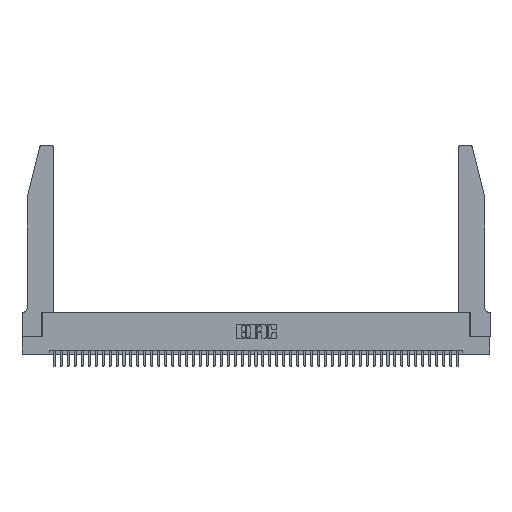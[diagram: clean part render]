
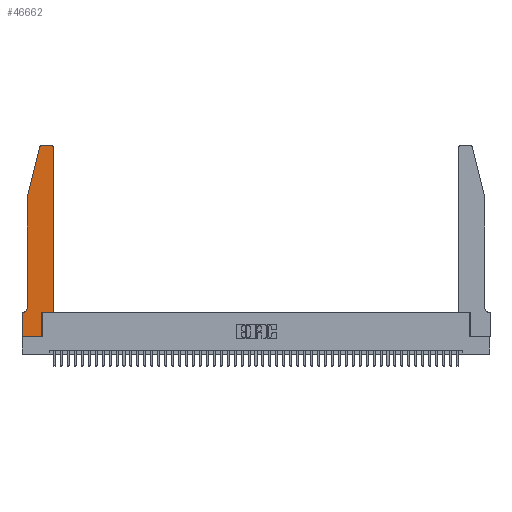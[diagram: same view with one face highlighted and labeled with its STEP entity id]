
A CAD part, top view. The second image highlights one B-rep face of the part: STEP entity #46662.
In plain terms, the highlighted planar face has unit normal (0, 0, 1).
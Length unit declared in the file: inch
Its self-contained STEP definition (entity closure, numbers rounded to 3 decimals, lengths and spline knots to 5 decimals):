
#1175 = AXIS2_PLACEMENT_3D ( 'NONE', #30477, #7696, #34262 ) ;
#1360 = EDGE_CURVE ( 'NONE', #37964, #4641, #27871, .T. ) ;
#1802 = VERTEX_POINT ( 'NONE', #13973 ) ;
#1859 = CARTESIAN_POINT ( 'NONE',  ( 0.0755, 2., 0.37 ) ) ;
#1992 = CARTESIAN_POINT ( 'NONE',  ( 0., 0., 0.37 ) ) ;
#2021 = DIRECTION ( 'NONE',  ( 0., 1., 0. ) ) ;
#2385 = DIRECTION ( 'NONE',  ( 0., -1., 0. ) ) ;
#2411 = EDGE_LOOP ( 'NONE', ( #35080, #6524, #41640, #19693, #6158, #15713, #20523, #47466, #19174, #46541, #48551, #15309 ) ) ;
#4641 = VERTEX_POINT ( 'NONE', #20457 ) ;
#5832 = CARTESIAN_POINT ( 'NONE',  ( 0.2865, 0.35, 0.37 ) ) ;
#6158 = ORIENTED_EDGE ( 'NONE', *, *, #45871, .T. ) ;
#6491 = VERTEX_POINT ( 'NONE', #12283 ) ;
#6518 = CARTESIAN_POINT ( 'NONE',  ( 0.2865, 0., 0.37 ) ) ;
#6524 = ORIENTED_EDGE ( 'NONE', *, *, #12069, .T. ) ;
#6620 = CIRCLE ( 'NONE', #1175, 0.07 ) ;
#7099 = CIRCLE ( 'NONE', #15949, 0.03 ) ;
#7696 = DIRECTION ( 'NONE',  ( 0., 0., -1. ) ) ;
#8002 = EDGE_CURVE ( 'NONE', #47248, #38260, #21926, .T. ) ;
#8680 = CARTESIAN_POINT ( 'NONE',  ( 0.25487, 2.72718, 0.37 ) ) ;
#8787 = LINE ( 'NONE', #15213, #39152 ) ;
#9561 = DIRECTION ( 'NONE',  ( 0., 0., 1. ) ) ;
#11467 = VERTEX_POINT ( 'NONE', #20448 ) ;
#12069 = EDGE_CURVE ( 'NONE', #30801, #13946, #47593, .T. ) ;
#12283 = CARTESIAN_POINT ( 'NONE',  ( 0.4205, 2.75, 0.37 ) ) ;
#12477 = CARTESIAN_POINT ( 'NONE',  ( 0.4205, 2.72, 0.37 ) ) ;
#13946 = VERTEX_POINT ( 'NONE', #8680 ) ;
#13973 = CARTESIAN_POINT ( 'NONE',  ( 0., 0.35, 0.37 ) ) ;
#14581 = AXIS2_PLACEMENT_3D ( 'NONE', #16002, #46081, #23686 ) ;
#14727 = LINE ( 'NONE', #1859, #43635 ) ;
#15213 = CARTESIAN_POINT ( 'NONE',  ( 0.2605, 2.75, 0.37 ) ) ;
#15309 = ORIENTED_EDGE ( 'NONE', *, *, #34329, .T. ) ;
#15360 = EDGE_CURVE ( 'NONE', #4641, #11467, #21247, .T. ) ;
#15378 = VERTEX_POINT ( 'NONE', #26697 ) ;
#15713 = ORIENTED_EDGE ( 'NONE', *, *, #29901, .T. ) ;
#15949 = AXIS2_PLACEMENT_3D ( 'NONE', #12477, #38962, #16351 ) ;
#16002 = CARTESIAN_POINT ( 'NONE',  ( 0., 0.35, 0.37 ) ) ;
#16351 = DIRECTION ( 'NONE',  ( 1., 0., 0. ) ) ;
#17013 = DIRECTION ( 'NONE',  ( -0.239, -0.971, 0. ) ) ;
#18178 = VERTEX_POINT ( 'NONE', #44987 ) ;
#18852 = DIRECTION ( 'NONE',  ( 0., 1., 0. ) ) ;
#19037 = DIRECTION ( 'NONE',  ( -1., 0., 0. ) ) ;
#19174 = ORIENTED_EDGE ( 'NONE', *, *, #48269, .T. ) ;
#19693 = ORIENTED_EDGE ( 'NONE', *, *, #43758, .T. ) ;
#20448 = CARTESIAN_POINT ( 'NONE',  ( 0.4505, 2.72, 0.37 ) ) ;
#20457 = CARTESIAN_POINT ( 'NONE',  ( 0.4505, 0.35, 0.37 ) ) ;
#20523 = ORIENTED_EDGE ( 'NONE', *, *, #46788, .T. ) ;
#20741 = VECTOR ( 'NONE', #36001, 39.37008 ) ;
#21167 = FACE_OUTER_BOUND ( 'NONE', #2411, .T. ) ;
#21247 = LINE ( 'NONE', #37838, #31309 ) ;
#21910 = CARTESIAN_POINT ( 'NONE',  ( 0.0755, 0.35, 0.37 ) ) ;
#21926 = LINE ( 'NONE', #1992, #20741 ) ;
#23614 = LINE ( 'NONE', #43894, #32454 ) ;
#23686 = DIRECTION ( 'NONE',  ( 1., 0., 0. ) ) ;
#24168 = CARTESIAN_POINT ( 'NONE',  ( 0., 0., 0.37 ) ) ;
#24680 = CARTESIAN_POINT ( 'NONE',  ( 0.0755, 0.42, 0.37 ) ) ;
#24793 = VECTOR ( 'NONE', #40813, 39.37008 ) ;
#25909 = AXIS2_PLACEMENT_3D ( 'NONE', #32343, #9561, #36102 ) ;
#26522 = LINE ( 'NONE', #24168, #46381 ) ;
#26685 = VECTOR ( 'NONE', #38451, 39.37008 ) ;
#26697 = CARTESIAN_POINT ( 'NONE',  ( 0.0755, 2., 0.37 ) ) ;
#27871 = LINE ( 'NONE', #30909, #26685 ) ;
#29475 = LINE ( 'NONE', #21910, #24793 ) ;
#29901 = EDGE_CURVE ( 'NONE', #18178, #1802, #29475, .T. ) ;
#30477 = CARTESIAN_POINT ( 'NONE',  ( 0.0055, 0.42, 0.37 ) ) ;
#30801 = VERTEX_POINT ( 'NONE', #31080 ) ;
#30909 = CARTESIAN_POINT ( 'NONE',  ( 0.4505, 0.35, 0.37 ) ) ;
#31080 = CARTESIAN_POINT ( 'NONE',  ( 0.284, 2.75, 0.37 ) ) ;
#31309 = VECTOR ( 'NONE', #18852, 39.37008 ) ;
#31566 = DIRECTION ( 'NONE',  ( 0., -1., 0. ) ) ;
#31655 = LINE ( 'NONE', #5832, #40444 ) ;
#32343 = CARTESIAN_POINT ( 'NONE',  ( 0.284, 2.72, 0.37 ) ) ;
#32454 = VECTOR ( 'NONE', #2385, 39.37008 ) ;
#32978 = EDGE_CURVE ( 'NONE', #6491, #30801, #8787, .T. ) ;
#33901 = VERTEX_POINT ( 'NONE', #24680 ) ;
#34262 = DIRECTION ( 'NONE',  ( -1., 0., 0. ) ) ;
#34329 = EDGE_CURVE ( 'NONE', #11467, #6491, #7099, .T. ) ;
#35080 = ORIENTED_EDGE ( 'NONE', *, *, #32978, .T. ) ;
#36001 = DIRECTION ( 'NONE',  ( 1., 0., 0. ) ) ;
#36102 = DIRECTION ( 'NONE',  ( 1., 0., 0. ) ) ;
#36408 = EDGE_CURVE ( 'NONE', #13946, #15378, #14727, .T. ) ;
#37838 = CARTESIAN_POINT ( 'NONE',  ( 0.4505, 0.35, 0.37 ) ) ;
#37964 = VERTEX_POINT ( 'NONE', #42455 ) ;
#38067 = CARTESIAN_POINT ( 'NONE',  ( 0., 0., 0.37 ) ) ;
#38260 = VERTEX_POINT ( 'NONE', #6518 ) ;
#38451 = DIRECTION ( 'NONE',  ( 1., 0., 0. ) ) ;
#38618 = PLANE ( 'NONE',  #14581 ) ;
#38962 = DIRECTION ( 'NONE',  ( 0., 0., 1. ) ) ;
#39152 = VECTOR ( 'NONE', #19037, 39.37008 ) ;
#40444 = VECTOR ( 'NONE', #2021, 39.37008 ) ;
#40813 = DIRECTION ( 'NONE',  ( -1., 0., 0. ) ) ;
#41640 = ORIENTED_EDGE ( 'NONE', *, *, #36408, .T. ) ;
#42455 = CARTESIAN_POINT ( 'NONE',  ( 0.2865, 0.35, 0.37 ) ) ;
#43635 = VECTOR ( 'NONE', #17013, 39.37008 ) ;
#43758 = EDGE_CURVE ( 'NONE', #15378, #33901, #23614, .T. ) ;
#43894 = CARTESIAN_POINT ( 'NONE',  ( 0.0755, 2., 0.37 ) ) ;
#44987 = CARTESIAN_POINT ( 'NONE',  ( 0.0055, 0.35, 0.37 ) ) ;
#45871 = EDGE_CURVE ( 'NONE', #33901, #18178, #6620, .T. ) ;
#46081 = DIRECTION ( 'NONE',  ( 0., 0., 1. ) ) ;
#46381 = VECTOR ( 'NONE', #31566, 39.37008 ) ;
#46541 = ORIENTED_EDGE ( 'NONE', *, *, #1360, .T. ) ;
#46662 = ADVANCED_FACE ( 'NONE', ( #21167 ), #38618, .T. ) ;
#46788 = EDGE_CURVE ( 'NONE', #1802, #47248, #26522, .T. ) ;
#47248 = VERTEX_POINT ( 'NONE', #38067 ) ;
#47466 = ORIENTED_EDGE ( 'NONE', *, *, #8002, .T. ) ;
#47593 = CIRCLE ( 'NONE', #25909, 0.03 ) ;
#48269 = EDGE_CURVE ( 'NONE', #38260, #37964, #31655, .T. ) ;
#48551 = ORIENTED_EDGE ( 'NONE', *, *, #15360, .T. ) ;
